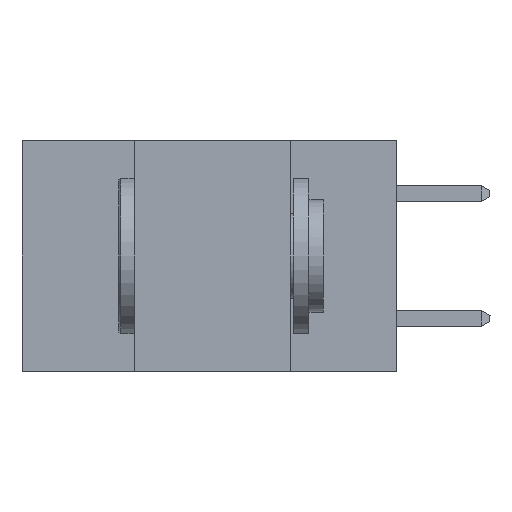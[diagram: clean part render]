
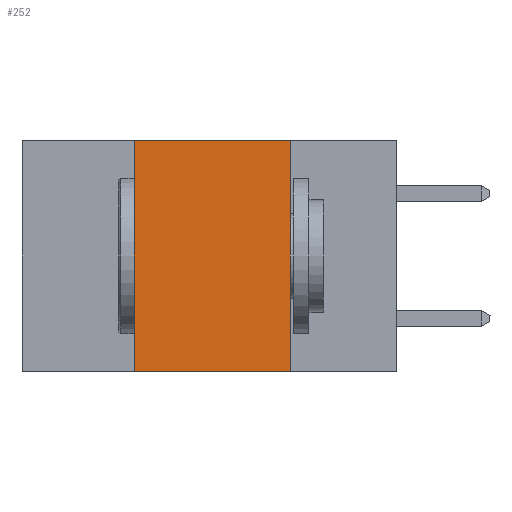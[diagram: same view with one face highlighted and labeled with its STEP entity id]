
A CAD part, left-side view. The second image highlights one B-rep face of the part: STEP entity #252.
In plain terms, the highlighted planar face has unit normal (-1, 0, 0).
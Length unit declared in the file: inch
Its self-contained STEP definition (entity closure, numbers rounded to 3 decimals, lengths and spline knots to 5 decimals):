
#252 = ADVANCED_FACE ( 'NONE', ( #6187 ), #14692, .F. ) ;
#524 = CARTESIAN_POINT ( 'NONE',  ( 0., 0.6, -0.37 ) ) ;
#942 = ORIENTED_EDGE ( 'NONE', *, *, #3717, .F. ) ;
#1299 = CARTESIAN_POINT ( 'NONE',  ( 0., 0.42, -0.37 ) ) ;
#1341 = VECTOR ( 'NONE', #9320, 39.37008 ) ;
#1811 = EDGE_CURVE ( 'NONE', #4723, #7802, #5739, .T. ) ;
#2941 = ORIENTED_EDGE ( 'NONE', *, *, #11317, .T. ) ;
#3011 = VERTEX_POINT ( 'NONE', #7929 ) ;
#3153 = CARTESIAN_POINT ( 'NONE',  ( 0., 0.17, 0. ) ) ;
#3287 = EDGE_LOOP ( 'NONE', ( #942, #9609, #8566, #2941 ) ) ;
#3717 = EDGE_CURVE ( 'NONE', #11172, #3011, #6081, .T. ) ;
#3803 = DIRECTION ( 'NONE',  ( 0., -1., 0. ) ) ;
#4472 = CARTESIAN_POINT ( 'NONE',  ( 0., 0.42, 0. ) ) ;
#4662 = DIRECTION ( 'NONE',  ( 0., 0., -1. ) ) ;
#4723 = VERTEX_POINT ( 'NONE', #1299 ) ;
#5491 = CARTESIAN_POINT ( 'NONE',  ( 0., 0.17, 0. ) ) ;
#5552 = DIRECTION ( 'NONE',  ( 0., 0., -1. ) ) ;
#5739 = LINE ( 'NONE', #4472, #1341 ) ;
#6081 = LINE ( 'NONE', #3153, #13239 ) ;
#6187 = FACE_OUTER_BOUND ( 'NONE', #3287, .T. ) ;
#6190 = LINE ( 'NONE', #524, #14697 ) ;
#7802 = VERTEX_POINT ( 'NONE', #10373 ) ;
#7929 = CARTESIAN_POINT ( 'NONE',  ( 0., 0.17, -0.37 ) ) ;
#8566 = ORIENTED_EDGE ( 'NONE', *, *, #1811, .F. ) ;
#8945 = VECTOR ( 'NONE', #3803, 39.37008 ) ;
#9320 = DIRECTION ( 'NONE',  ( 0., 0., 1. ) ) ;
#9609 = ORIENTED_EDGE ( 'NONE', *, *, #14326, .F. ) ;
#9907 = AXIS2_PLACEMENT_3D ( 'NONE', #13400, #11030, #4662 ) ;
#10373 = CARTESIAN_POINT ( 'NONE',  ( 0., 0.42, 0. ) ) ;
#10412 = DIRECTION ( 'NONE',  ( 0., -1., 0. ) ) ;
#11030 = DIRECTION ( 'NONE',  ( 1., 0., 0. ) ) ;
#11172 = VERTEX_POINT ( 'NONE', #5491 ) ;
#11317 = EDGE_CURVE ( 'NONE', #4723, #3011, #6190, .T. ) ;
#11848 = CARTESIAN_POINT ( 'NONE',  ( 0., 0.6, 0. ) ) ;
#13239 = VECTOR ( 'NONE', #5552, 39.37008 ) ;
#13400 = CARTESIAN_POINT ( 'NONE',  ( 0., 0.6, 0. ) ) ;
#14326 = EDGE_CURVE ( 'NONE', #7802, #11172, #15881, .T. ) ;
#14692 = PLANE ( 'NONE',  #9907 ) ;
#14697 = VECTOR ( 'NONE', #10412, 39.37008 ) ;
#15881 = LINE ( 'NONE', #11848, #8945 ) ;
